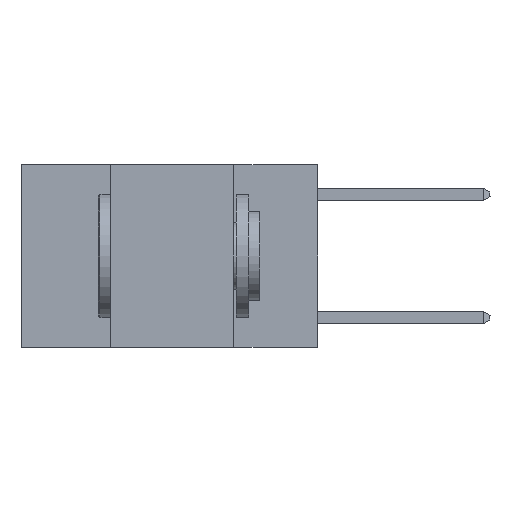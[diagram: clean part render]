
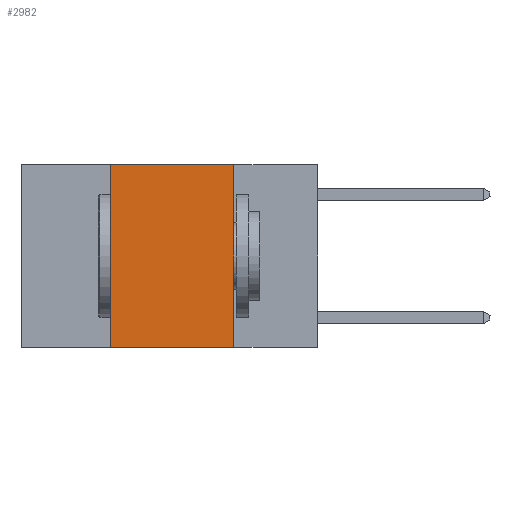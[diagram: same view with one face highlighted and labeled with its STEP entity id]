
A CAD part, left-side view. The second image highlights one B-rep face of the part: STEP entity #2982.
In plain terms, the highlighted planar face has unit normal (-1, 0, 0).
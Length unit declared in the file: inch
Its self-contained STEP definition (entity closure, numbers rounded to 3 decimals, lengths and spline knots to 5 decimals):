
#565 = EDGE_CURVE ( 'NONE', #15322, #9636, #928, .T. ) ;
#928 = LINE ( 'NONE', #5608, #14651 ) ;
#1638 = AXIS2_PLACEMENT_3D ( 'NONE', #15716, #22182, #24866 ) ;
#1966 = CARTESIAN_POINT ( 'NONE',  ( 0., 0.42, 0. ) ) ;
#2029 = CARTESIAN_POINT ( 'NONE',  ( 0., 0.6, 0. ) ) ;
#2982 = ADVANCED_FACE ( 'NONE', ( #27120 ), #22031, .F. ) ;
#3289 = CARTESIAN_POINT ( 'NONE',  ( 0., 0.6, -0.37 ) ) ;
#4956 = VECTOR ( 'NONE', #11877, 39.37008 ) ;
#5608 = CARTESIAN_POINT ( 'NONE',  ( 0., 0.17, 0. ) ) ;
#8841 = CARTESIAN_POINT ( 'NONE',  ( 0., 0.42, 0. ) ) ;
#9636 = VERTEX_POINT ( 'NONE', #12578 ) ;
#9717 = ORIENTED_EDGE ( 'NONE', *, *, #565, .F. ) ;
#11158 = EDGE_CURVE ( 'NONE', #15229, #15322, #27421, .T. ) ;
#11544 = LINE ( 'NONE', #8841, #23256 ) ;
#11877 = DIRECTION ( 'NONE',  ( 0., -1., 0. ) ) ;
#12336 = CARTESIAN_POINT ( 'NONE',  ( 0., 0.17, 0. ) ) ;
#12578 = CARTESIAN_POINT ( 'NONE',  ( 0., 0.17, -0.37 ) ) ;
#13191 = ORIENTED_EDGE ( 'NONE', *, *, #11158, .F. ) ;
#14651 = VECTOR ( 'NONE', #25891, 39.37008 ) ;
#14722 = LINE ( 'NONE', #3289, #4956 ) ;
#15229 = VERTEX_POINT ( 'NONE', #1966 ) ;
#15322 = VERTEX_POINT ( 'NONE', #12336 ) ;
#15576 = DIRECTION ( 'NONE',  ( 0., -1., 0. ) ) ;
#15716 = CARTESIAN_POINT ( 'NONE',  ( 0., 0.6, 0. ) ) ;
#17132 = EDGE_CURVE ( 'NONE', #22650, #9636, #14722, .T. ) ;
#17263 = VECTOR ( 'NONE', #15576, 39.37008 ) ;
#18306 = DIRECTION ( 'NONE',  ( 0., 0., 1. ) ) ;
#18681 = EDGE_CURVE ( 'NONE', #22650, #15229, #11544, .T. ) ;
#20392 = ORIENTED_EDGE ( 'NONE', *, *, #18681, .F. ) ;
#20748 = ORIENTED_EDGE ( 'NONE', *, *, #17132, .T. ) ;
#22031 = PLANE ( 'NONE',  #1638 ) ;
#22182 = DIRECTION ( 'NONE',  ( 1., 0., 0. ) ) ;
#22650 = VERTEX_POINT ( 'NONE', #27989 ) ;
#23256 = VECTOR ( 'NONE', #18306, 39.37008 ) ;
#24866 = DIRECTION ( 'NONE',  ( 0., 0., -1. ) ) ;
#25891 = DIRECTION ( 'NONE',  ( 0., 0., -1. ) ) ;
#27004 = EDGE_LOOP ( 'NONE', ( #9717, #13191, #20392, #20748 ) ) ;
#27120 = FACE_OUTER_BOUND ( 'NONE', #27004, .T. ) ;
#27421 = LINE ( 'NONE', #2029, #17263 ) ;
#27989 = CARTESIAN_POINT ( 'NONE',  ( 0., 0.42, -0.37 ) ) ;
